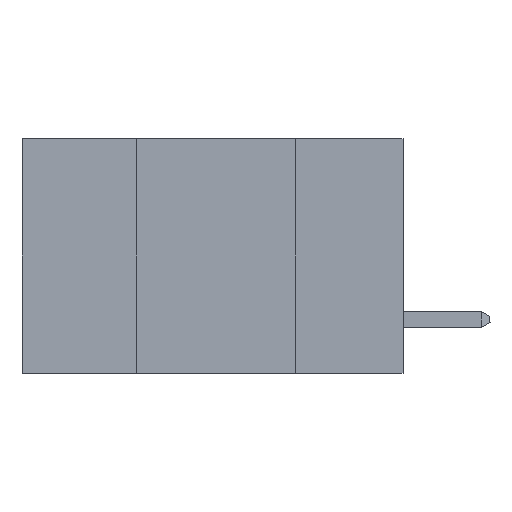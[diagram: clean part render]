
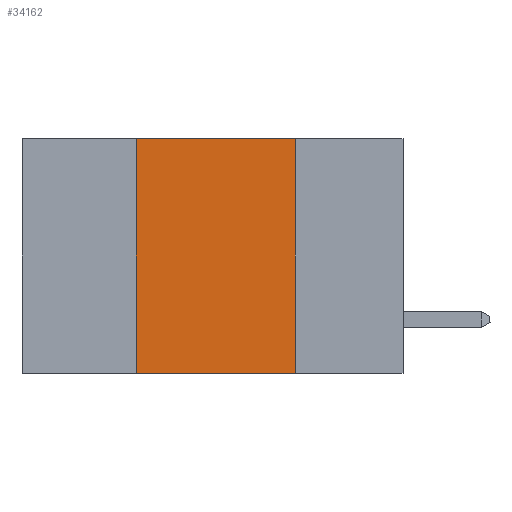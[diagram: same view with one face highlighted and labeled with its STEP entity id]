
A CAD part, left-side view. The second image highlights one B-rep face of the part: STEP entity #34162.
In plain terms, the highlighted planar face has unit normal (-1, 0, 0).
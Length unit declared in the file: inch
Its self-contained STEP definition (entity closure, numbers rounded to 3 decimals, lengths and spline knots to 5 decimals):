
#654 = CARTESIAN_POINT ( 'NONE',  ( 0., 0.6, 0. ) ) ;
#1064 = CARTESIAN_POINT ( 'NONE',  ( 0., 0.17, 0. ) ) ;
#1165 = EDGE_CURVE ( 'NONE', #22644, #23685, #37794, .T. ) ;
#2086 = VERTEX_POINT ( 'NONE', #26014 ) ;
#2867 = CARTESIAN_POINT ( 'NONE',  ( 0., 0.17, -0.37 ) ) ;
#3677 = DIRECTION ( 'NONE',  ( 1., 0., 0. ) ) ;
#5204 = LINE ( 'NONE', #10640, #12367 ) ;
#6041 = DIRECTION ( 'NONE',  ( 0., -1., 0. ) ) ;
#8881 = CARTESIAN_POINT ( 'NONE',  ( 0., 0.6, -0.37 ) ) ;
#9757 = EDGE_CURVE ( 'NONE', #2086, #22644, #16514, .T. ) ;
#10640 = CARTESIAN_POINT ( 'NONE',  ( 0., 0.42, 0. ) ) ;
#10789 = DIRECTION ( 'NONE',  ( 0., 0., 1. ) ) ;
#11209 = EDGE_CURVE ( 'NONE', #32730, #2086, #5204, .T. ) ;
#12367 = VECTOR ( 'NONE', #10789, 39.37008 ) ;
#15763 = EDGE_LOOP ( 'NONE', ( #21476, #27772, #25407, #37082 ) ) ;
#15850 = VECTOR ( 'NONE', #6041, 39.37008 ) ;
#16514 = LINE ( 'NONE', #39560, #20601 ) ;
#16775 = DIRECTION ( 'NONE',  ( 0., 0., -1. ) ) ;
#18346 = LINE ( 'NONE', #8881, #15850 ) ;
#20232 = AXIS2_PLACEMENT_3D ( 'NONE', #654, #3677, #26589 ) ;
#20601 = VECTOR ( 'NONE', #30008, 39.37008 ) ;
#21476 = ORIENTED_EDGE ( 'NONE', *, *, #1165, .F. ) ;
#22644 = VERTEX_POINT ( 'NONE', #1064 ) ;
#23685 = VERTEX_POINT ( 'NONE', #2867 ) ;
#25407 = ORIENTED_EDGE ( 'NONE', *, *, #11209, .F. ) ;
#26014 = CARTESIAN_POINT ( 'NONE',  ( 0., 0.42, 0. ) ) ;
#26462 = CARTESIAN_POINT ( 'NONE',  ( 0., 0.42, -0.37 ) ) ;
#26589 = DIRECTION ( 'NONE',  ( 0., 0., -1. ) ) ;
#27772 = ORIENTED_EDGE ( 'NONE', *, *, #9757, .F. ) ;
#30008 = DIRECTION ( 'NONE',  ( 0., -1., 0. ) ) ;
#32730 = VERTEX_POINT ( 'NONE', #26462 ) ;
#32846 = CARTESIAN_POINT ( 'NONE',  ( 0., 0.17, 0. ) ) ;
#33314 = FACE_OUTER_BOUND ( 'NONE', #15763, .T. ) ;
#34162 = ADVANCED_FACE ( 'NONE', ( #33314 ), #39240, .F. ) ;
#36237 = VECTOR ( 'NONE', #16775, 39.37008 ) ;
#37082 = ORIENTED_EDGE ( 'NONE', *, *, #40033, .T. ) ;
#37794 = LINE ( 'NONE', #32846, #36237 ) ;
#39240 = PLANE ( 'NONE',  #20232 ) ;
#39560 = CARTESIAN_POINT ( 'NONE',  ( 0., 0.6, 0. ) ) ;
#40033 = EDGE_CURVE ( 'NONE', #32730, #23685, #18346, .T. ) ;
